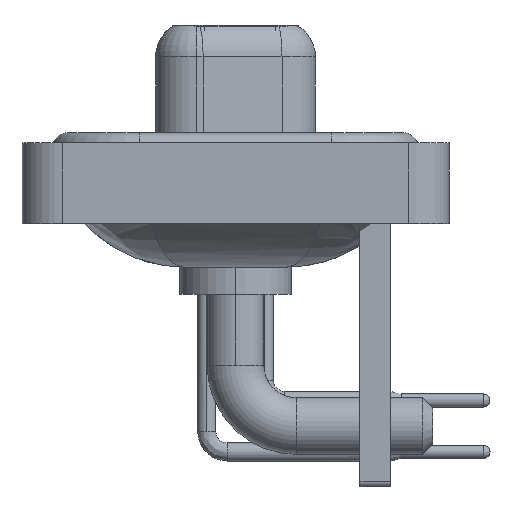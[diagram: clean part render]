
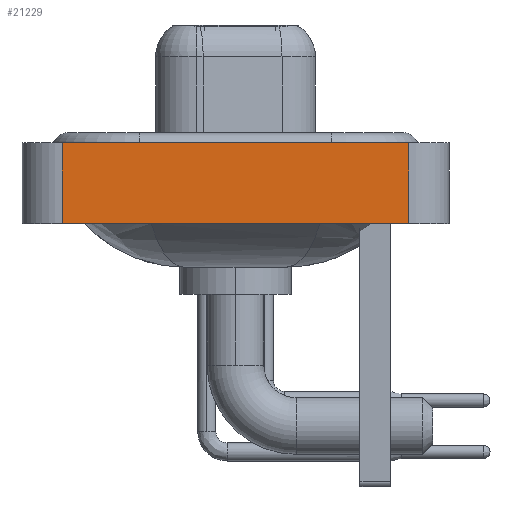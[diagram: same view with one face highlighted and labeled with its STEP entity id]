
A CAD part, left-side view. The second image highlights one B-rep face of the part: STEP entity #21229.
In plain terms, the highlighted planar face has unit normal (-1, 0, 0).
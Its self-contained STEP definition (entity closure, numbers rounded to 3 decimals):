
#1772 = LINE ( 'NONE', #12579, #12403 ) ;
#1928 = ORIENTED_EDGE ( 'NONE', *, *, #16199, .T. ) ;
#3080 = CARTESIAN_POINT ( 'NONE',  ( -7.35, -8.55, -3.6 ) ) ;
#3187 = DIRECTION ( 'NONE',  ( 0., 0., 1. ) ) ;
#3580 = EDGE_LOOP ( 'NONE', ( #19809, #6068, #13312, #1928 ) ) ;
#4876 = FACE_OUTER_BOUND ( 'NONE', #3580, .T. ) ;
#6068 = ORIENTED_EDGE ( 'NONE', *, *, #8826, .F. ) ;
#6240 = CARTESIAN_POINT ( 'NONE',  ( -7.35, 8.55, -3.6 ) ) ;
#7532 = LINE ( 'NONE', #18194, #10559 ) ;
#7682 = LINE ( 'NONE', #16821, #22751 ) ;
#8573 = DIRECTION ( 'NONE',  ( 0., 0., 1. ) ) ;
#8826 = EDGE_CURVE ( 'NONE', #10048, #19967, #7682, .T. ) ;
#9428 = VECTOR ( 'NONE', #8573, 1000. ) ;
#9490 = AXIS2_PLACEMENT_3D ( 'NONE', #3080, #10034, #3187 ) ;
#9861 = CARTESIAN_POINT ( 'NONE',  ( -7.35, -8.55, -3.6 ) ) ;
#10034 = DIRECTION ( 'NONE',  ( -1., 0., 0. ) ) ;
#10048 = VERTEX_POINT ( 'NONE', #18260 ) ;
#10559 = VECTOR ( 'NONE', #14880, 1000. ) ;
#10689 = EDGE_CURVE ( 'NONE', #20173, #10048, #1772, .T. ) ;
#12397 = LINE ( 'NONE', #17799, #9428 ) ;
#12403 = VECTOR ( 'NONE', #16420, 1000. ) ;
#12579 = CARTESIAN_POINT ( 'NONE',  ( -7.35, 8.55, -3.6 ) ) ;
#13312 = ORIENTED_EDGE ( 'NONE', *, *, #10689, .F. ) ;
#14880 = DIRECTION ( 'NONE',  ( 0., -1., 0. ) ) ;
#16199 = EDGE_CURVE ( 'NONE', #20173, #20151, #7532, .T. ) ;
#16420 = DIRECTION ( 'NONE',  ( 0., 0., 1. ) ) ;
#16821 = CARTESIAN_POINT ( 'NONE',  ( -7.35, -8.55, 0.4 ) ) ;
#17051 = DIRECTION ( 'NONE',  ( 0., -1., 0. ) ) ;
#17697 = PLANE ( 'NONE',  #9490 ) ;
#17799 = CARTESIAN_POINT ( 'NONE',  ( -7.35, -8.55, -3.6 ) ) ;
#18194 = CARTESIAN_POINT ( 'NONE',  ( -7.35, -8.55, -3.6 ) ) ;
#18260 = CARTESIAN_POINT ( 'NONE',  ( -7.35, 8.55, 0.4 ) ) ;
#19451 = EDGE_CURVE ( 'NONE', #20151, #19967, #12397, .T. ) ;
#19809 = ORIENTED_EDGE ( 'NONE', *, *, #19451, .T. ) ;
#19967 = VERTEX_POINT ( 'NONE', #21336 ) ;
#20151 = VERTEX_POINT ( 'NONE', #9861 ) ;
#20173 = VERTEX_POINT ( 'NONE', #6240 ) ;
#21229 = ADVANCED_FACE ( 'NONE', ( #4876 ), #17697, .T. ) ;
#21336 = CARTESIAN_POINT ( 'NONE',  ( -7.35, -8.55, 0.4 ) ) ;
#22751 = VECTOR ( 'NONE', #17051, 1000. ) ;
